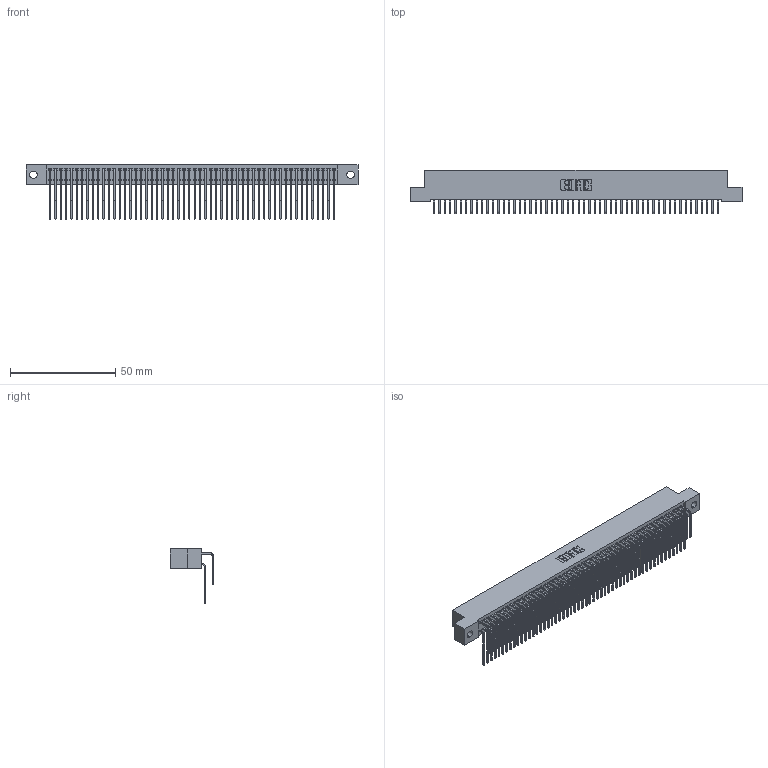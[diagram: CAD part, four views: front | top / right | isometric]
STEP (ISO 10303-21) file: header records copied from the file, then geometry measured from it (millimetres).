
FILE_DESCRIPTION (( 'STEP AP203' ), '1' );
FILE_NAME ('392-108-559-202.STEP', '2019-10-09T23:26:19', ( '' ), ( '' ), 'SwSTEP 2.0', 'SolidWorks 2016', '' );
FILE_SCHEMA (( 'CONFIG_CONTROL_DESIGN' ));
Length unit declared in the file: inch
Products named in the file (4): 342 Part_.128 Slot; 345-292-001_558 559 Tail - 1; 345-292-001_559 Tail - 2; 392-108-559-202
Assembly tree (109 placements, depth 2):
  392-108-559-202
    342 Part_.128 Slot
    345-292-001_558 559 Tail - 1  x54
    345-292-001_559 Tail - 2  x54
Bounding box: 157.48 x 20.64 x 25.78 mm (x, y, z)
Volume: 14777.2 mm3; surface area: 26927.1 mm2
Topology: 109 solids, 109 shells, 5946 faces, 17699 edges, 11654 vertices
Faces by surface type: plane 4174, cylinder 1772
Entity records: 34975 total; most frequent: CARTESIAN_POINT 5833, ORIENTED_EDGE 5718, DIRECTION 4943, EDGE_CURVE 2859, LINE 2691, VECTOR 2691, VERTEX_POINT 1902, AXIS2_PLACEMENT_3D 1126
